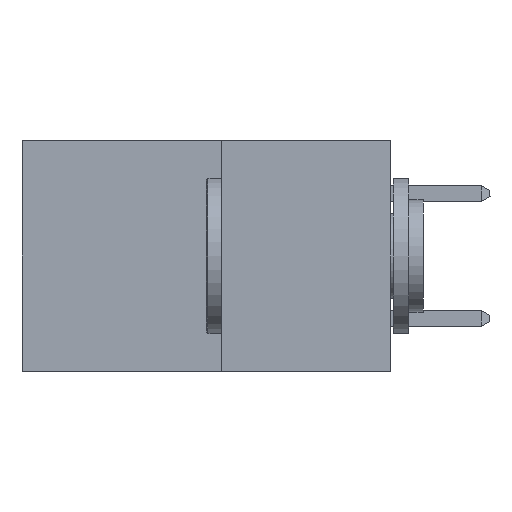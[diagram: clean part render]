
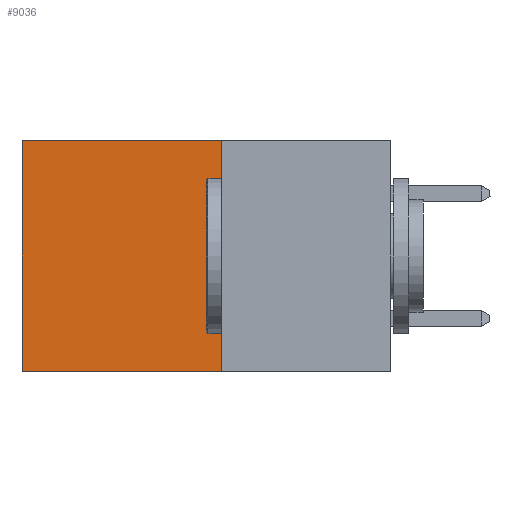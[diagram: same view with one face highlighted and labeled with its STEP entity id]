
A CAD part, left-side view. The second image highlights one B-rep face of the part: STEP entity #9036.
In plain terms, the highlighted planar face has unit normal (-1, 0, 0).
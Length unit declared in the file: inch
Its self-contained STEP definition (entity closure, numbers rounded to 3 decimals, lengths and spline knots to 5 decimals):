
#355 = DIRECTION ( 'NONE',  ( 0., 0., -1. ) ) ;
#1178 = CARTESIAN_POINT ( 'NONE',  ( 0.277, 0.27, 0. ) ) ;
#1338 = CARTESIAN_POINT ( 'NONE',  ( 0.277, 0.27, 0. ) ) ;
#1533 = ORIENTED_EDGE ( 'NONE', *, *, #17415, .T. ) ;
#1672 = DIRECTION ( 'NONE',  ( 1., 0., 0. ) ) ;
#2102 = VERTEX_POINT ( 'NONE', #1338 ) ;
#2199 = ORIENTED_EDGE ( 'NONE', *, *, #13264, .T. ) ;
#2361 = VECTOR ( 'NONE', #10970, 39.37008 ) ;
#2754 = CARTESIAN_POINT ( 'NONE',  ( 0.277, 0.59, -0.37 ) ) ;
#3061 = CARTESIAN_POINT ( 'NONE',  ( 0.277, 0.59, 0. ) ) ;
#3724 = ORIENTED_EDGE ( 'NONE', *, *, #15262, .F. ) ;
#4230 = VERTEX_POINT ( 'NONE', #13713 ) ;
#4554 = FACE_OUTER_BOUND ( 'NONE', #8455, .T. ) ;
#4629 = EDGE_CURVE ( 'NONE', #4230, #7500, #16971, .T. ) ;
#4766 = LINE ( 'NONE', #1178, #2361 ) ;
#5014 = AXIS2_PLACEMENT_3D ( 'NONE', #5801, #1672, #11474 ) ;
#5604 = DIRECTION ( 'NONE',  ( 0., 0., -1. ) ) ;
#5801 = CARTESIAN_POINT ( 'NONE',  ( 0.277, 0.27, -0.37 ) ) ;
#5992 = VECTOR ( 'NONE', #15684, 39.37008 ) ;
#7500 = VERTEX_POINT ( 'NONE', #2754 ) ;
#8455 = EDGE_LOOP ( 'NONE', ( #1533, #16259, #3724, #2199 ) ) ;
#8956 = LINE ( 'NONE', #15609, #15893 ) ;
#9036 = ADVANCED_FACE ( 'NONE', ( #4554 ), #15514, .F. ) ;
#10970 = DIRECTION ( 'NONE',  ( 0., 1., 0. ) ) ;
#11474 = DIRECTION ( 'NONE',  ( 0., 0., -1. ) ) ;
#12590 = CARTESIAN_POINT ( 'NONE',  ( 0.277, 0.27, -0.37 ) ) ;
#12595 = VECTOR ( 'NONE', #5604, 39.37008 ) ;
#13264 = EDGE_CURVE ( 'NONE', #2102, #16594, #4766, .T. ) ;
#13713 = CARTESIAN_POINT ( 'NONE',  ( 0.277, 0.27, -0.37 ) ) ;
#15262 = EDGE_CURVE ( 'NONE', #2102, #4230, #17374, .T. ) ;
#15514 = PLANE ( 'NONE',  #5014 ) ;
#15609 = CARTESIAN_POINT ( 'NONE',  ( 0.277, 0.59, -0.37 ) ) ;
#15684 = DIRECTION ( 'NONE',  ( 0., 1., 0. ) ) ;
#15893 = VECTOR ( 'NONE', #355, 39.37008 ) ;
#16259 = ORIENTED_EDGE ( 'NONE', *, *, #4629, .F. ) ;
#16498 = CARTESIAN_POINT ( 'NONE',  ( 0.277, 0.27, -0.37 ) ) ;
#16594 = VERTEX_POINT ( 'NONE', #3061 ) ;
#16971 = LINE ( 'NONE', #16498, #5992 ) ;
#17374 = LINE ( 'NONE', #12590, #12595 ) ;
#17415 = EDGE_CURVE ( 'NONE', #16594, #7500, #8956, .T. ) ;
